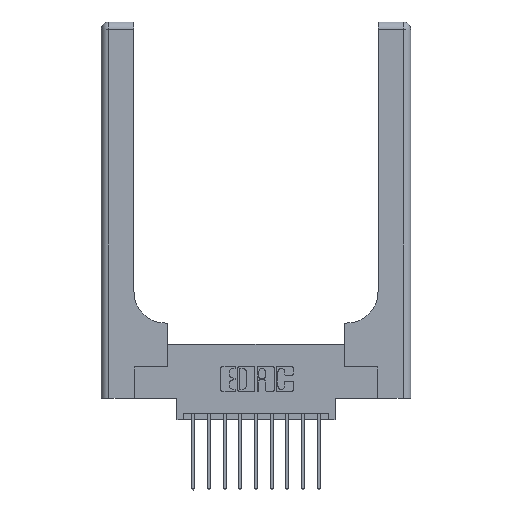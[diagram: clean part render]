
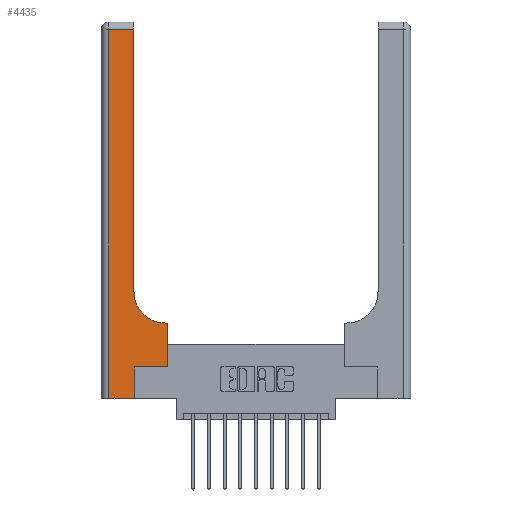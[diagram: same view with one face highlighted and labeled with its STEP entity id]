
A CAD part, top view. The second image highlights one B-rep face of the part: STEP entity #4435.
In plain terms, the highlighted planar face has unit normal (0, 0, 1).
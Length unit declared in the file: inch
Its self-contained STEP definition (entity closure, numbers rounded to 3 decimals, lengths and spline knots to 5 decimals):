
#218 = ORIENTED_EDGE ( 'NONE', *, *, #11186, .T. ) ;
#420 = DIRECTION ( 'NONE',  ( 1., 0., 0. ) ) ;
#623 = ORIENTED_EDGE ( 'NONE', *, *, #15656, .T. ) ;
#685 = CARTESIAN_POINT ( 'NONE',  ( 0.51, 0.85, 0.37 ) ) ;
#1000 = LINE ( 'NONE', #8158, #13507 ) ;
#1103 = CARTESIAN_POINT ( 'NONE',  ( 0.51, 0.6, 0.37 ) ) ;
#1394 = DIRECTION ( 'NONE',  ( -1., 0., 0. ) ) ;
#1429 = VECTOR ( 'NONE', #6018, 39.37008 ) ;
#1737 = AXIS2_PLACEMENT_3D ( 'NONE', #3778, #8654, #1394 ) ;
#1923 = DIRECTION ( 'NONE',  ( 1., 0., 0. ) ) ;
#2036 = AXIS2_PLACEMENT_3D ( 'NONE', #685, #9164, #1923 ) ;
#2412 = EDGE_CURVE ( 'NONE', #8327, #14434, #14460, .T. ) ;
#2787 = CARTESIAN_POINT ( 'NONE',  ( 0.26, 2.94, 0.37 ) ) ;
#2856 = LINE ( 'NONE', #5259, #15327 ) ;
#3336 = DIRECTION ( 'NONE',  ( 0., -1., 0. ) ) ;
#3583 = DIRECTION ( 'NONE',  ( -1., 0., 0. ) ) ;
#3724 = CARTESIAN_POINT ( 'NONE',  ( 0.528, 0.25, 0.37 ) ) ;
#3778 = CARTESIAN_POINT ( 'NONE',  ( 0., 3., 0.37 ) ) ;
#3949 = VECTOR ( 'NONE', #10983, 39.37008 ) ;
#4116 = CARTESIAN_POINT ( 'NONE',  ( 0.265, 0., 0.37 ) ) ;
#4135 = DIRECTION ( 'NONE',  ( -1., 0., 0. ) ) ;
#4435 = ADVANCED_FACE ( 'NONE', ( #6444 ), #7446, .F. ) ;
#4525 = VERTEX_POINT ( 'NONE', #6335 ) ;
#4793 = VECTOR ( 'NONE', #10350, 39.37008 ) ;
#5042 = CARTESIAN_POINT ( 'NONE',  ( 0.265, 0.25, 0.37 ) ) ;
#5259 = CARTESIAN_POINT ( 'NONE',  ( 0.265, 0.25, 0.37 ) ) ;
#5714 = ORIENTED_EDGE ( 'NONE', *, *, #7340, .T. ) ;
#5735 = ORIENTED_EDGE ( 'NONE', *, *, #2412, .T. ) ;
#5788 = CARTESIAN_POINT ( 'NONE',  ( 0.06, 0., 0.37 ) ) ;
#6018 = DIRECTION ( 'NONE',  ( 0., 1., 0. ) ) ;
#6335 = CARTESIAN_POINT ( 'NONE',  ( 0.528, 0.6, 0.37 ) ) ;
#6444 = FACE_OUTER_BOUND ( 'NONE', #9483, .T. ) ;
#6582 = VERTEX_POINT ( 'NONE', #14006 ) ;
#6917 = VERTEX_POINT ( 'NONE', #9612 ) ;
#7106 = CIRCLE ( 'NONE', #2036, 0.25 ) ;
#7340 = EDGE_CURVE ( 'NONE', #11931, #8731, #13559, .T. ) ;
#7440 = ORIENTED_EDGE ( 'NONE', *, *, #11024, .T. ) ;
#7446 = PLANE ( 'NONE',  #1737 ) ;
#7590 = EDGE_CURVE ( 'NONE', #8731, #6582, #10526, .T. ) ;
#7781 = VECTOR ( 'NONE', #8008, 39.37008 ) ;
#8008 = DIRECTION ( 'NONE',  ( 1., 0., 0. ) ) ;
#8158 = CARTESIAN_POINT ( 'NONE',  ( 0.06, 3., 0.37 ) ) ;
#8327 = VERTEX_POINT ( 'NONE', #4116 ) ;
#8375 = CARTESIAN_POINT ( 'NONE',  ( 0.26, 0.85, 0.37 ) ) ;
#8654 = DIRECTION ( 'NONE',  ( 0., 0., -1. ) ) ;
#8731 = VERTEX_POINT ( 'NONE', #2787 ) ;
#9164 = DIRECTION ( 'NONE',  ( 0., 0., -1. ) ) ;
#9483 = EDGE_LOOP ( 'NONE', ( #5714, #11181, #13303, #218, #5735, #7440, #12247, #12627, #623 ) ) ;
#9501 = VECTOR ( 'NONE', #3583, 39.37008 ) ;
#9612 = CARTESIAN_POINT ( 'NONE',  ( 0.528, 0.25, 0.37 ) ) ;
#10113 = EDGE_CURVE ( 'NONE', #6582, #14298, #1000, .T. ) ;
#10248 = LINE ( 'NONE', #15232, #7781 ) ;
#10266 = LINE ( 'NONE', #10844, #9501 ) ;
#10350 = DIRECTION ( 'NONE',  ( 0., 1., 0. ) ) ;
#10526 = LINE ( 'NONE', #12613, #13737 ) ;
#10791 = EDGE_CURVE ( 'NONE', #4525, #15320, #10266, .T. ) ;
#10844 = CARTESIAN_POINT ( 'NONE',  ( 0.26, 0.6, 0.37 ) ) ;
#10983 = DIRECTION ( 'NONE',  ( 0., 1., 0. ) ) ;
#11024 = EDGE_CURVE ( 'NONE', #14434, #6917, #2856, .T. ) ;
#11181 = ORIENTED_EDGE ( 'NONE', *, *, #7590, .T. ) ;
#11186 = EDGE_CURVE ( 'NONE', #14298, #8327, #10248, .T. ) ;
#11577 = CARTESIAN_POINT ( 'NONE',  ( 0.265, 0., 0.37 ) ) ;
#11931 = VERTEX_POINT ( 'NONE', #8375 ) ;
#12247 = ORIENTED_EDGE ( 'NONE', *, *, #12963, .T. ) ;
#12613 = CARTESIAN_POINT ( 'NONE',  ( 0., 2.94, 0.37 ) ) ;
#12627 = ORIENTED_EDGE ( 'NONE', *, *, #10791, .T. ) ;
#12963 = EDGE_CURVE ( 'NONE', #6917, #4525, #14371, .T. ) ;
#13255 = CARTESIAN_POINT ( 'NONE',  ( 0.26, 3., 0.37 ) ) ;
#13303 = ORIENTED_EDGE ( 'NONE', *, *, #10113, .T. ) ;
#13507 = VECTOR ( 'NONE', #3336, 39.37008 ) ;
#13559 = LINE ( 'NONE', #13255, #1429 ) ;
#13737 = VECTOR ( 'NONE', #4135, 39.37008 ) ;
#14006 = CARTESIAN_POINT ( 'NONE',  ( 0.06, 2.94, 0.37 ) ) ;
#14298 = VERTEX_POINT ( 'NONE', #5788 ) ;
#14371 = LINE ( 'NONE', #3724, #3949 ) ;
#14434 = VERTEX_POINT ( 'NONE', #5042 ) ;
#14460 = LINE ( 'NONE', #11577, #4793 ) ;
#15232 = CARTESIAN_POINT ( 'NONE',  ( 0., 0., 0.37 ) ) ;
#15320 = VERTEX_POINT ( 'NONE', #1103 ) ;
#15327 = VECTOR ( 'NONE', #420, 39.37008 ) ;
#15656 = EDGE_CURVE ( 'NONE', #15320, #11931, #7106, .T. ) ;
